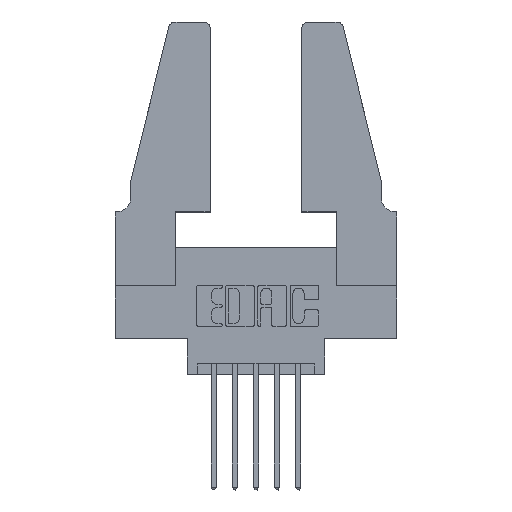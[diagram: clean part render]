
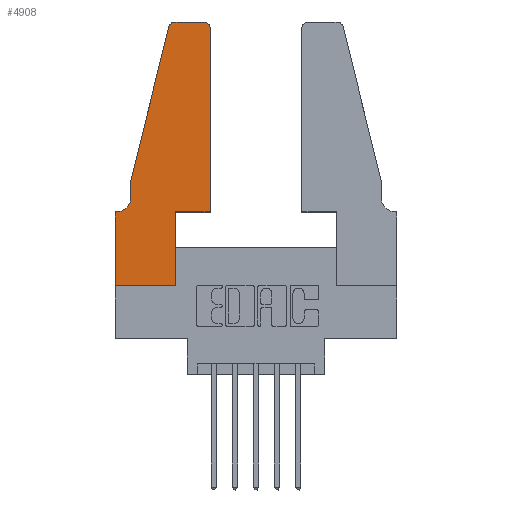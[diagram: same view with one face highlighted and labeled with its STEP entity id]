
A CAD part, top view. The second image highlights one B-rep face of the part: STEP entity #4908.
In plain terms, the highlighted planar face has unit normal (0, 0, 1).
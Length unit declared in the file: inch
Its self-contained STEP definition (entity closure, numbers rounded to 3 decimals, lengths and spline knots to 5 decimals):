
#57 = ORIENTED_EDGE ( 'NONE', *, *, #6576, .T. ) ;
#76 = LINE ( 'NONE', #1989, #8532 ) ;
#116 = ORIENTED_EDGE ( 'NONE', *, *, #2070, .T. ) ;
#276 = ORIENTED_EDGE ( 'NONE', *, *, #1702, .T. ) ;
#322 = EDGE_CURVE ( 'NONE', #7367, #7875, #2139, .T. ) ;
#497 = DIRECTION ( 'NONE',  ( 0., 0., 1. ) ) ;
#538 = VECTOR ( 'NONE', #4408, 39.37008 ) ;
#568 = LINE ( 'NONE', #6496, #5199 ) ;
#679 = LINE ( 'NONE', #5445, #9621 ) ;
#773 = CARTESIAN_POINT ( 'NONE',  ( 0.0755, 0.5, 0.37 ) ) ;
#1702 = EDGE_CURVE ( 'NONE', #6671, #7421, #568, .T. ) ;
#1725 = VERTEX_POINT ( 'NONE', #10063 ) ;
#1730 = DIRECTION ( 'NONE',  ( 1., 0., 0. ) ) ;
#1752 = DIRECTION ( 'NONE',  ( 0., 0., 1. ) ) ;
#1770 = CARTESIAN_POINT ( 'NONE',  ( 0.4205, 1.22, 0.37 ) ) ;
#1893 = EDGE_CURVE ( 'NONE', #10643, #6671, #7354, .T. ) ;
#1989 = CARTESIAN_POINT ( 'NONE',  ( 0.0755, 0.5, 0.37 ) ) ;
#2070 = EDGE_CURVE ( 'NONE', #4112, #7367, #3983, .T. ) ;
#2072 = DIRECTION ( 'NONE',  ( 1., 0., 0. ) ) ;
#2076 = DIRECTION ( 'NONE',  ( 0., 0., 1. ) ) ;
#2099 = CIRCLE ( 'NONE', #9991, 0.07 ) ;
#2109 = PLANE ( 'NONE',  #3280 ) ;
#2139 = LINE ( 'NONE', #3795, #11047 ) ;
#2251 = CARTESIAN_POINT ( 'NONE',  ( 0., 0.35, 0.37 ) ) ;
#2289 = ORIENTED_EDGE ( 'NONE', *, *, #4950, .T. ) ;
#2367 = LINE ( 'NONE', #7906, #6714 ) ;
#2387 = ORIENTED_EDGE ( 'NONE', *, *, #322, .T. ) ;
#2394 = CARTESIAN_POINT ( 'NONE',  ( 0., 0., 0.37 ) ) ;
#2509 = EDGE_CURVE ( 'NONE', #3130, #1725, #3420, .T. ) ;
#2778 = EDGE_CURVE ( 'NONE', #6520, #4112, #679, .T. ) ;
#2821 = DIRECTION ( 'NONE',  ( 1., 0., 0. ) ) ;
#2830 = CARTESIAN_POINT ( 'NONE',  ( 0.2865, 0., 0.37 ) ) ;
#2923 = VERTEX_POINT ( 'NONE', #3458 ) ;
#3019 = VECTOR ( 'NONE', #2821, 39.37008 ) ;
#3130 = VERTEX_POINT ( 'NONE', #11127 ) ;
#3280 = AXIS2_PLACEMENT_3D ( 'NONE', #2251, #2076, #2072 ) ;
#3373 = CARTESIAN_POINT ( 'NONE',  ( 0.4505, 1.22, 0.37 ) ) ;
#3420 = LINE ( 'NONE', #9511, #10561 ) ;
#3458 = CARTESIAN_POINT ( 'NONE',  ( 0.0755, 0.42, 0.37 ) ) ;
#3702 = CARTESIAN_POINT ( 'NONE',  ( 0.25487, 1.22718, 0.37 ) ) ;
#3795 = CARTESIAN_POINT ( 'NONE',  ( 0.0755, 0.5, 0.37 ) ) ;
#3983 = CIRCLE ( 'NONE', #4082, 0.03 ) ;
#4082 = AXIS2_PLACEMENT_3D ( 'NONE', #6409, #497, #9340 ) ;
#4112 = VERTEX_POINT ( 'NONE', #6406 ) ;
#4181 = CARTESIAN_POINT ( 'NONE',  ( 0.4505, 0.35, 0.37 ) ) ;
#4371 = CARTESIAN_POINT ( 'NONE',  ( 0., 0., 0.37 ) ) ;
#4408 = DIRECTION ( 'NONE',  ( 1., 0., 0. ) ) ;
#4458 = AXIS2_PLACEMENT_3D ( 'NONE', #1770, #1752, #1730 ) ;
#4469 = CIRCLE ( 'NONE', #4458, 0.03 ) ;
#4544 = DIRECTION ( 'NONE',  ( 0., 0., -1. ) ) ;
#4735 = FACE_OUTER_BOUND ( 'NONE', #5385, .T. ) ;
#4816 = VERTEX_POINT ( 'NONE', #2830 ) ;
#4908 = ADVANCED_FACE ( 'NONE', ( #4735 ), #2109, .T. ) ;
#4950 = EDGE_CURVE ( 'NONE', #7421, #6520, #4469, .T. ) ;
#5199 = VECTOR ( 'NONE', #6475, 39.37008 ) ;
#5228 = ORIENTED_EDGE ( 'NONE', *, *, #7164, .T. ) ;
#5268 = DIRECTION ( 'NONE',  ( -1., 0., 0. ) ) ;
#5278 = CARTESIAN_POINT ( 'NONE',  ( 0.0055, 0.42, 0.37 ) ) ;
#5385 = EDGE_LOOP ( 'NONE', ( #7122, #116, #2387, #10155, #7514, #6852, #9635, #5228, #57, #10188, #276, #2289 ) ) ;
#5445 = CARTESIAN_POINT ( 'NONE',  ( 0.2605, 1.25, 0.37 ) ) ;
#5784 = DIRECTION ( 'NONE',  ( 0., 1., 0. ) ) ;
#5973 = CARTESIAN_POINT ( 'NONE',  ( 0.2865, 0.35, 0.37 ) ) ;
#6291 = EDGE_CURVE ( 'NONE', #1725, #7580, #2367, .T. ) ;
#6302 = EDGE_CURVE ( 'NONE', #2923, #3130, #2099, .T. ) ;
#6324 = DIRECTION ( 'NONE',  ( 0., -1., 0. ) ) ;
#6406 = CARTESIAN_POINT ( 'NONE',  ( 0.284, 1.25, 0.37 ) ) ;
#6409 = CARTESIAN_POINT ( 'NONE',  ( 0.284, 1.22, 0.37 ) ) ;
#6448 = CARTESIAN_POINT ( 'NONE',  ( 0.4205, 1.25, 0.37 ) ) ;
#6475 = DIRECTION ( 'NONE',  ( 0., 1., 0. ) ) ;
#6496 = CARTESIAN_POINT ( 'NONE',  ( 0.4505, 0.35, 0.37 ) ) ;
#6520 = VERTEX_POINT ( 'NONE', #6448 ) ;
#6576 = EDGE_CURVE ( 'NONE', #4816, #10643, #11134, .T. ) ;
#6671 = VERTEX_POINT ( 'NONE', #10156 ) ;
#6714 = VECTOR ( 'NONE', #8972, 39.37008 ) ;
#6852 = ORIENTED_EDGE ( 'NONE', *, *, #2509, .T. ) ;
#7122 = ORIENTED_EDGE ( 'NONE', *, *, #2778, .T. ) ;
#7164 = EDGE_CURVE ( 'NONE', #7580, #4816, #7204, .T. ) ;
#7204 = LINE ( 'NONE', #4371, #538 ) ;
#7354 = LINE ( 'NONE', #4181, #3019 ) ;
#7367 = VERTEX_POINT ( 'NONE', #3702 ) ;
#7421 = VERTEX_POINT ( 'NONE', #3373 ) ;
#7514 = ORIENTED_EDGE ( 'NONE', *, *, #6302, .T. ) ;
#7580 = VERTEX_POINT ( 'NONE', #2394 ) ;
#7875 = VERTEX_POINT ( 'NONE', #773 ) ;
#7906 = CARTESIAN_POINT ( 'NONE',  ( 0., 0., 0.37 ) ) ;
#8168 = DIRECTION ( 'NONE',  ( -0.239, -0.971, 0. ) ) ;
#8532 = VECTOR ( 'NONE', #6324, 39.37008 ) ;
#8624 = EDGE_CURVE ( 'NONE', #7875, #2923, #76, .T. ) ;
#8885 = VECTOR ( 'NONE', #5784, 39.37008 ) ;
#8972 = DIRECTION ( 'NONE',  ( 0., -1., 0. ) ) ;
#9245 = DIRECTION ( 'NONE',  ( -1., 0., 0. ) ) ;
#9340 = DIRECTION ( 'NONE',  ( 1., 0., 0. ) ) ;
#9511 = CARTESIAN_POINT ( 'NONE',  ( 0.0755, 0.35, 0.37 ) ) ;
#9621 = VECTOR ( 'NONE', #5268, 39.37008 ) ;
#9635 = ORIENTED_EDGE ( 'NONE', *, *, #6291, .T. ) ;
#9991 = AXIS2_PLACEMENT_3D ( 'NONE', #5278, #4544, #10269 ) ;
#10063 = CARTESIAN_POINT ( 'NONE',  ( 0., 0.35, 0.37 ) ) ;
#10114 = CARTESIAN_POINT ( 'NONE',  ( 0.2865, 0.35, 0.37 ) ) ;
#10155 = ORIENTED_EDGE ( 'NONE', *, *, #8624, .T. ) ;
#10156 = CARTESIAN_POINT ( 'NONE',  ( 0.4505, 0.35, 0.37 ) ) ;
#10188 = ORIENTED_EDGE ( 'NONE', *, *, #1893, .T. ) ;
#10269 = DIRECTION ( 'NONE',  ( -1., 0., 0. ) ) ;
#10561 = VECTOR ( 'NONE', #9245, 39.37008 ) ;
#10643 = VERTEX_POINT ( 'NONE', #10114 ) ;
#11047 = VECTOR ( 'NONE', #8168, 39.37008 ) ;
#11127 = CARTESIAN_POINT ( 'NONE',  ( 0.0055, 0.35, 0.37 ) ) ;
#11134 = LINE ( 'NONE', #5973, #8885 ) ;
